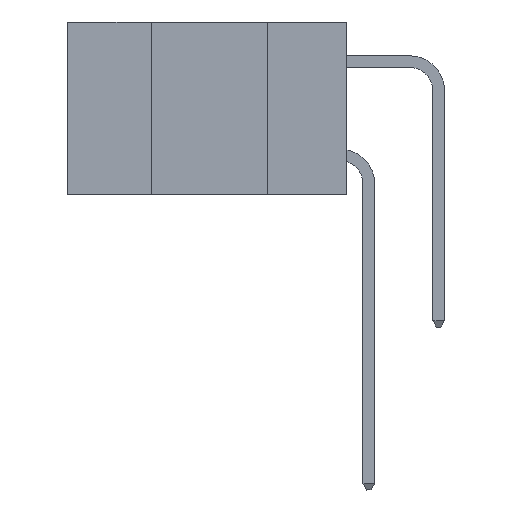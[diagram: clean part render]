
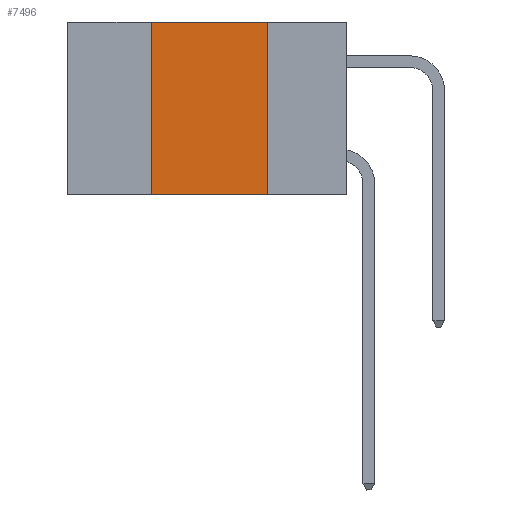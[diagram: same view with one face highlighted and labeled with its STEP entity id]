
A CAD part, left-side view. The second image highlights one B-rep face of the part: STEP entity #7496.
In plain terms, the highlighted planar face has unit normal (-1, 0, 0).
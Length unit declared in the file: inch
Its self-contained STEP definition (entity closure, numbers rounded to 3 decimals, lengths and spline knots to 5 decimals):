
#484 = ORIENTED_EDGE ( 'NONE', *, *, #9065, .F. ) ;
#2209 = EDGE_CURVE ( 'NONE', #14219, #14281, #9221, .T. ) ;
#2589 = LINE ( 'NONE', #24629, #13989 ) ;
#2951 = FACE_OUTER_BOUND ( 'NONE', #24501, .T. ) ;
#4498 = DIRECTION ( 'NONE',  ( 0., 0., -1. ) ) ;
#4664 = LINE ( 'NONE', #25165, #7818 ) ;
#7395 = ORIENTED_EDGE ( 'NONE', *, *, #32002, .F. ) ;
#7496 = ADVANCED_FACE ( 'NONE', ( #2951 ), #28606, .F. ) ;
#7667 = VERTEX_POINT ( 'NONE', #30118 ) ;
#7757 = LINE ( 'NONE', #17057, #16013 ) ;
#7818 = VECTOR ( 'NONE', #30265, 39.37008 ) ;
#8196 = EDGE_CURVE ( 'NONE', #7667, #22369, #2589, .T. ) ;
#9065 = EDGE_CURVE ( 'NONE', #14281, #22369, #7757, .T. ) ;
#9221 = LINE ( 'NONE', #23055, #16696 ) ;
#13989 = VECTOR ( 'NONE', #32076, 39.37008 ) ;
#14219 = VERTEX_POINT ( 'NONE', #16815 ) ;
#14281 = VERTEX_POINT ( 'NONE', #30375 ) ;
#15273 = DIRECTION ( 'NONE',  ( 0., -1., 0. ) ) ;
#15294 = AXIS2_PLACEMENT_3D ( 'NONE', #31114, #23693, #21270 ) ;
#16013 = VECTOR ( 'NONE', #4498, 39.37008 ) ;
#16696 = VECTOR ( 'NONE', #15273, 39.37008 ) ;
#16815 = CARTESIAN_POINT ( 'NONE',  ( 0., 0.42, 0. ) ) ;
#17057 = CARTESIAN_POINT ( 'NONE',  ( 0., 0.17, 0. ) ) ;
#17198 = ORIENTED_EDGE ( 'NONE', *, *, #2209, .F. ) ;
#21270 = DIRECTION ( 'NONE',  ( 0., 0., -1. ) ) ;
#22369 = VERTEX_POINT ( 'NONE', #29378 ) ;
#23055 = CARTESIAN_POINT ( 'NONE',  ( 0., 0.6, 0. ) ) ;
#23693 = DIRECTION ( 'NONE',  ( 1., 0., 0. ) ) ;
#24501 = EDGE_LOOP ( 'NONE', ( #484, #17198, #7395, #29116 ) ) ;
#24629 = CARTESIAN_POINT ( 'NONE',  ( 0., 0.6, -0.37 ) ) ;
#25165 = CARTESIAN_POINT ( 'NONE',  ( 0., 0.42, 0. ) ) ;
#28606 = PLANE ( 'NONE',  #15294 ) ;
#29116 = ORIENTED_EDGE ( 'NONE', *, *, #8196, .T. ) ;
#29378 = CARTESIAN_POINT ( 'NONE',  ( 0., 0.17, -0.37 ) ) ;
#30118 = CARTESIAN_POINT ( 'NONE',  ( 0., 0.42, -0.37 ) ) ;
#30265 = DIRECTION ( 'NONE',  ( 0., 0., 1. ) ) ;
#30375 = CARTESIAN_POINT ( 'NONE',  ( 0., 0.17, 0. ) ) ;
#31114 = CARTESIAN_POINT ( 'NONE',  ( 0., 0.6, 0. ) ) ;
#32002 = EDGE_CURVE ( 'NONE', #7667, #14219, #4664, .T. ) ;
#32076 = DIRECTION ( 'NONE',  ( 0., -1., 0. ) ) ;
